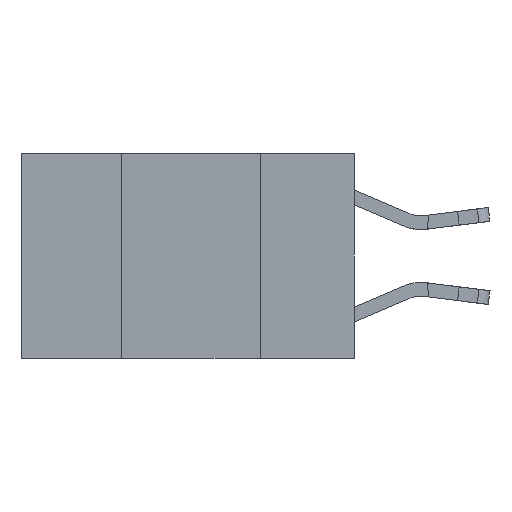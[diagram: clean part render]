
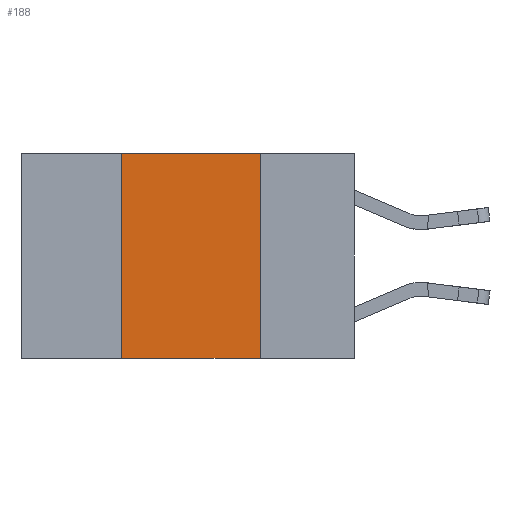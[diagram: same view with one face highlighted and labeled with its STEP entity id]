
A CAD part, left-side view. The second image highlights one B-rep face of the part: STEP entity #188.
In plain terms, the highlighted planar face has unit normal (-1, 0, 0).
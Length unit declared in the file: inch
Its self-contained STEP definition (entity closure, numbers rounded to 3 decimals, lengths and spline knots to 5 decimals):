
#188 = ADVANCED_FACE ( 'NONE', ( #16592 ), #2494, .F. ) ;
#1959 = EDGE_CURVE ( 'NONE', #6920, #18048, #5723, .T. ) ;
#2007 = CARTESIAN_POINT ( 'NONE',  ( 0., 0.42, 0. ) ) ;
#2494 = PLANE ( 'NONE',  #9643 ) ;
#2878 = LINE ( 'NONE', #15824, #17618 ) ;
#3736 = LINE ( 'NONE', #2007, #13957 ) ;
#4117 = DIRECTION ( 'NONE',  ( 0., -1., 0. ) ) ;
#4339 = EDGE_LOOP ( 'NONE', ( #7158, #23099, #8946, #10755 ) ) ;
#4449 = DIRECTION ( 'NONE',  ( 1., 0., 0. ) ) ;
#4612 = VECTOR ( 'NONE', #7427, 39.37008 ) ;
#5723 = LINE ( 'NONE', #17553, #10213 ) ;
#6109 = CARTESIAN_POINT ( 'NONE',  ( 0., 0.42, 0. ) ) ;
#6920 = VERTEX_POINT ( 'NONE', #7483 ) ;
#7158 = ORIENTED_EDGE ( 'NONE', *, *, #12307, .F. ) ;
#7427 = DIRECTION ( 'NONE',  ( 0., -1., 0. ) ) ;
#7483 = CARTESIAN_POINT ( 'NONE',  ( 0., 0.42, -0.37 ) ) ;
#7562 = CARTESIAN_POINT ( 'NONE',  ( 0., 0.17, -0.37 ) ) ;
#8412 = EDGE_CURVE ( 'NONE', #6920, #16925, #3736, .T. ) ;
#8946 = ORIENTED_EDGE ( 'NONE', *, *, #8412, .F. ) ;
#9643 = AXIS2_PLACEMENT_3D ( 'NONE', #15954, #4449, #17875 ) ;
#10213 = VECTOR ( 'NONE', #4117, 39.37008 ) ;
#10755 = ORIENTED_EDGE ( 'NONE', *, *, #1959, .T. ) ;
#12307 = EDGE_CURVE ( 'NONE', #24185, #18048, #2878, .T. ) ;
#13534 = DIRECTION ( 'NONE',  ( 0., 0., 1. ) ) ;
#13957 = VECTOR ( 'NONE', #13534, 39.37008 ) ;
#15063 = CARTESIAN_POINT ( 'NONE',  ( 0., 0.6, 0. ) ) ;
#15824 = CARTESIAN_POINT ( 'NONE',  ( 0., 0.17, 0. ) ) ;
#15954 = CARTESIAN_POINT ( 'NONE',  ( 0., 0.6, 0. ) ) ;
#16592 = FACE_OUTER_BOUND ( 'NONE', #4339, .T. ) ;
#16925 = VERTEX_POINT ( 'NONE', #6109 ) ;
#17383 = EDGE_CURVE ( 'NONE', #16925, #24185, #19935, .T. ) ;
#17553 = CARTESIAN_POINT ( 'NONE',  ( 0., 0.6, -0.37 ) ) ;
#17618 = VECTOR ( 'NONE', #19700, 39.37008 ) ;
#17875 = DIRECTION ( 'NONE',  ( 0., 0., -1. ) ) ;
#18048 = VERTEX_POINT ( 'NONE', #7562 ) ;
#19700 = DIRECTION ( 'NONE',  ( 0., 0., -1. ) ) ;
#19935 = LINE ( 'NONE', #15063, #4612 ) ;
#23099 = ORIENTED_EDGE ( 'NONE', *, *, #17383, .F. ) ;
#23545 = CARTESIAN_POINT ( 'NONE',  ( 0., 0.17, 0. ) ) ;
#24185 = VERTEX_POINT ( 'NONE', #23545 ) ;
